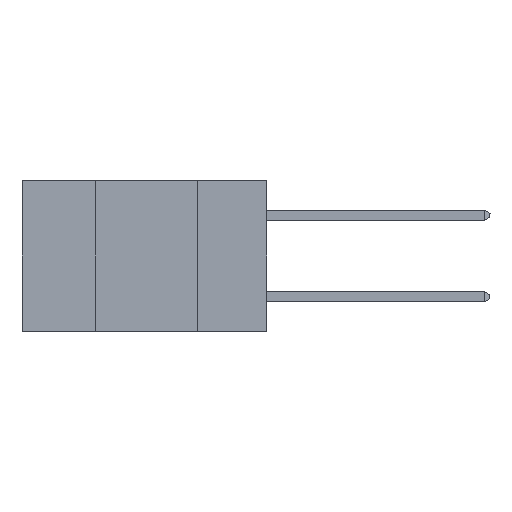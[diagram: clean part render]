
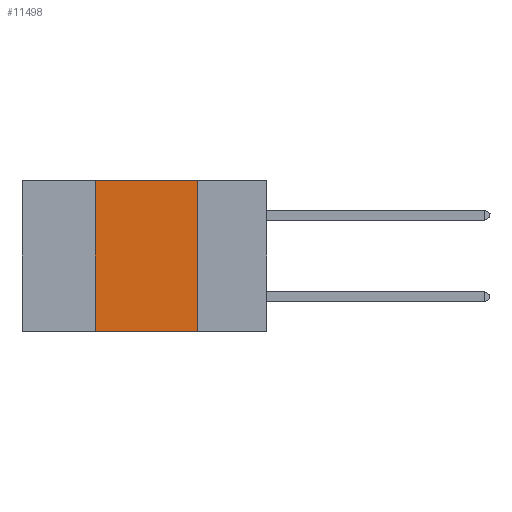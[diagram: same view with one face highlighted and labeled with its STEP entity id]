
A CAD part, left-side view. The second image highlights one B-rep face of the part: STEP entity #11498.
In plain terms, the highlighted planar face has unit normal (-1, 0, 0).
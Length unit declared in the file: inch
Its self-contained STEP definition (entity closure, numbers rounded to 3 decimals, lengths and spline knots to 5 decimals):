
#144 = CARTESIAN_POINT ( 'NONE',  ( 0., 0.42, 0. ) ) ;
#172 = DIRECTION ( 'NONE',  ( 0., -1., 0. ) ) ;
#287 = CARTESIAN_POINT ( 'NONE',  ( 0., 0.6, 0. ) ) ;
#494 = ORIENTED_EDGE ( 'NONE', *, *, #11520, .F. ) ;
#847 = CARTESIAN_POINT ( 'NONE',  ( 0., 0.6, -0.37 ) ) ;
#2448 = VECTOR ( 'NONE', #172, 39.37008 ) ;
#2905 = ORIENTED_EDGE ( 'NONE', *, *, #9590, .F. ) ;
#3481 = CARTESIAN_POINT ( 'NONE',  ( 0., 0.17, -0.37 ) ) ;
#3684 = EDGE_CURVE ( 'NONE', #15031, #14119, #6284, .T. ) ;
#3747 = CARTESIAN_POINT ( 'NONE',  ( 0., 0.42, 0. ) ) ;
#3971 = AXIS2_PLACEMENT_3D ( 'NONE', #287, #4452, #15531 ) ;
#4452 = DIRECTION ( 'NONE',  ( 1., 0., 0. ) ) ;
#4468 = CARTESIAN_POINT ( 'NONE',  ( 0., 0.42, -0.37 ) ) ;
#4991 = LINE ( 'NONE', #14356, #14124 ) ;
#5006 = CARTESIAN_POINT ( 'NONE',  ( 0., 0.6, 0. ) ) ;
#5679 = DIRECTION ( 'NONE',  ( 0., 0., 1. ) ) ;
#6284 = LINE ( 'NONE', #847, #2448 ) ;
#7177 = FACE_OUTER_BOUND ( 'NONE', #12176, .T. ) ;
#8447 = EDGE_CURVE ( 'NONE', #16680, #9905, #9359, .T. ) ;
#9296 = ORIENTED_EDGE ( 'NONE', *, *, #3684, .T. ) ;
#9359 = LINE ( 'NONE', #5006, #13551 ) ;
#9590 = EDGE_CURVE ( 'NONE', #15031, #16680, #12579, .T. ) ;
#9905 = VERTEX_POINT ( 'NONE', #14438 ) ;
#11498 = ADVANCED_FACE ( 'NONE', ( #7177 ), #12721, .F. ) ;
#11520 = EDGE_CURVE ( 'NONE', #9905, #14119, #4991, .T. ) ;
#11554 = VECTOR ( 'NONE', #5679, 39.37008 ) ;
#12176 = EDGE_LOOP ( 'NONE', ( #494, #16444, #2905, #9296 ) ) ;
#12579 = LINE ( 'NONE', #144, #11554 ) ;
#12721 = PLANE ( 'NONE',  #3971 ) ;
#13551 = VECTOR ( 'NONE', #16270, 39.37008 ) ;
#14119 = VERTEX_POINT ( 'NONE', #3481 ) ;
#14124 = VECTOR ( 'NONE', #14705, 39.37008 ) ;
#14356 = CARTESIAN_POINT ( 'NONE',  ( 0., 0.17, 0. ) ) ;
#14438 = CARTESIAN_POINT ( 'NONE',  ( 0., 0.17, 0. ) ) ;
#14705 = DIRECTION ( 'NONE',  ( 0., 0., -1. ) ) ;
#15031 = VERTEX_POINT ( 'NONE', #4468 ) ;
#15531 = DIRECTION ( 'NONE',  ( 0., 0., -1. ) ) ;
#16270 = DIRECTION ( 'NONE',  ( 0., -1., 0. ) ) ;
#16444 = ORIENTED_EDGE ( 'NONE', *, *, #8447, .F. ) ;
#16680 = VERTEX_POINT ( 'NONE', #3747 ) ;
